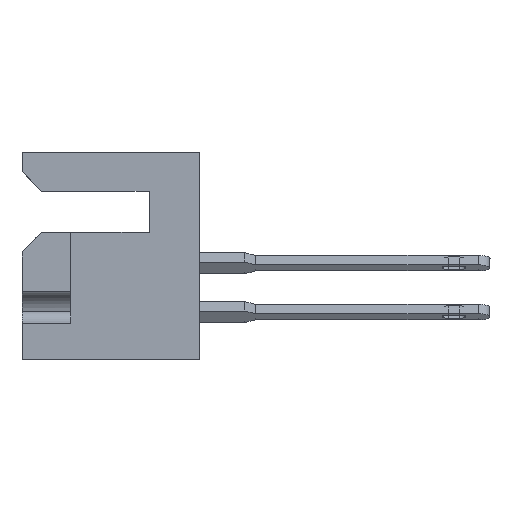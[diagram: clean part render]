
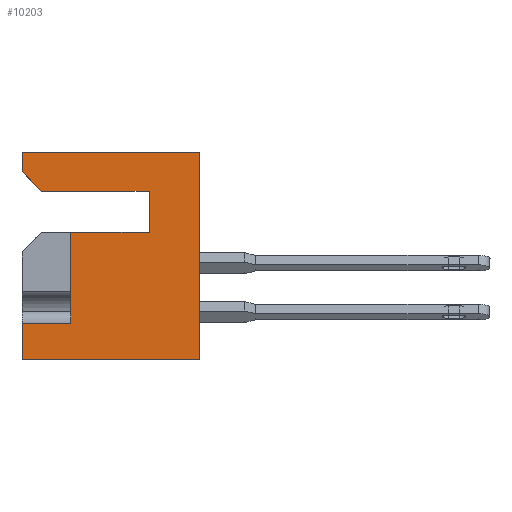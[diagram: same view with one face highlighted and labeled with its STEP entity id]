
A CAD part, left-side view. The second image highlights one B-rep face of the part: STEP entity #10203.
In plain terms, the highlighted planar face has unit normal (-1, 0, 0).
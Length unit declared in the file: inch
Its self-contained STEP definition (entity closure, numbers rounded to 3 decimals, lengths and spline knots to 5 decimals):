
#196 = VECTOR ( 'NONE', #16317, 39.37008 ) ;
#318 = DIRECTION ( 'NONE',  ( 0., -0.707, -0.707 ) ) ;
#600 = CARTESIAN_POINT ( 'NONE',  ( 0., 0.453, -0.437 ) ) ;
#619 = CARTESIAN_POINT ( 'NONE',  ( 0., 0.128, -0.1 ) ) ;
#1051 = DIRECTION ( 'NONE',  ( 0., 1., 0. ) ) ;
#1158 = ORIENTED_EDGE ( 'NONE', *, *, #29404, .F. ) ;
#1740 = EDGE_CURVE ( 'NONE', #29804, #2285, #30222, .T. ) ;
#2200 = EDGE_CURVE ( 'NONE', #2285, #3240, #10678, .T. ) ;
#2285 = VERTEX_POINT ( 'NONE', #9911 ) ;
#2516 = CARTESIAN_POINT ( 'NONE',  ( 0., 0.403, -0.1 ) ) ;
#2696 = LINE ( 'NONE', #619, #21012 ) ;
#3166 = DIRECTION ( 'NONE',  ( 0., 0., 1. ) ) ;
#3240 = VERTEX_POINT ( 'NONE', #20967 ) ;
#3398 = DIRECTION ( 'NONE',  ( 0., -1., 0. ) ) ;
#3488 = CARTESIAN_POINT ( 'NONE',  ( 0., 0.453, 0. ) ) ;
#3806 = ORIENTED_EDGE ( 'NONE', *, *, #1740, .T. ) ;
#4312 = CARTESIAN_POINT ( 'NONE',  ( 0., 0.453, -0.531 ) ) ;
#4360 = LINE ( 'NONE', #29978, #6949 ) ;
#5384 = CARTESIAN_POINT ( 'NONE',  ( 0., 0.453, -0.05 ) ) ;
#5457 = DIRECTION ( 'NONE',  ( 0., 0., 1. ) ) ;
#5610 = EDGE_CURVE ( 'NONE', #9739, #10014, #2696, .T. ) ;
#5795 = DIRECTION ( 'NONE',  ( 0., 1., 0. ) ) ;
#5845 = LINE ( 'NONE', #22413, #17781 ) ;
#6382 = EDGE_CURVE ( 'NONE', #22043, #27314, #6722, .T. ) ;
#6520 = LINE ( 'NONE', #18295, #196 ) ;
#6701 = CARTESIAN_POINT ( 'NONE',  ( 0., 0.128, -0.1 ) ) ;
#6722 = LINE ( 'NONE', #3488, #17491 ) ;
#6949 = VECTOR ( 'NONE', #1051, 39.37008 ) ;
#8115 = ORIENTED_EDGE ( 'NONE', *, *, #6382, .F. ) ;
#8143 = EDGE_CURVE ( 'NONE', #27314, #3240, #26451, .T. ) ;
#8195 = EDGE_CURVE ( 'NONE', #22358, #12789, #5845, .T. ) ;
#9115 = ORIENTED_EDGE ( 'NONE', *, *, #26209, .T. ) ;
#9739 = VERTEX_POINT ( 'NONE', #14934 ) ;
#9799 = DIRECTION ( 'NONE',  ( 0., 0., -1. ) ) ;
#9810 = CARTESIAN_POINT ( 'NONE',  ( 0., 0., 0. ) ) ;
#9911 = CARTESIAN_POINT ( 'NONE',  ( 0., 0., -0.531 ) ) ;
#10014 = VERTEX_POINT ( 'NONE', #6701 ) ;
#10203 = ADVANCED_FACE ( 'NONE', ( #15813 ), #17280, .F. ) ;
#10678 = LINE ( 'NONE', #9810, #23476 ) ;
#10777 = EDGE_CURVE ( 'NONE', #22043, #25842, #23697, .T. ) ;
#11663 = VECTOR ( 'NONE', #318, 39.37008 ) ;
#12358 = CARTESIAN_POINT ( 'NONE',  ( 0., 0.453, -0.531 ) ) ;
#12447 = ORIENTED_EDGE ( 'NONE', *, *, #5610, .F. ) ;
#12789 = VERTEX_POINT ( 'NONE', #17185 ) ;
#13010 = EDGE_CURVE ( 'NONE', #10014, #25842, #4360, .T. ) ;
#13811 = EDGE_CURVE ( 'NONE', #22358, #18755, #6520, .T. ) ;
#14658 = EDGE_LOOP ( 'NONE', ( #23924, #1158, #3806, #28747, #28792, #8115, #25415, #25661, #12447, #9115, #21869 ) ) ;
#14934 = CARTESIAN_POINT ( 'NONE',  ( 0., 0.128, -0.205 ) ) ;
#15813 = FACE_OUTER_BOUND ( 'NONE', #14658, .T. ) ;
#16317 = DIRECTION ( 'NONE',  ( 0., 1., 0. ) ) ;
#16990 = DIRECTION ( 'NONE',  ( 1., 0., 0. ) ) ;
#17185 = CARTESIAN_POINT ( 'NONE',  ( 0., 0.328, -0.205 ) ) ;
#17280 = PLANE ( 'NONE',  #22154 ) ;
#17491 = VECTOR ( 'NONE', #24609, 39.37008 ) ;
#17781 = VECTOR ( 'NONE', #17960, 39.37008 ) ;
#17811 = VECTOR ( 'NONE', #21823, 39.37008 ) ;
#17960 = DIRECTION ( 'NONE',  ( 0., 0., 1. ) ) ;
#18295 = CARTESIAN_POINT ( 'NONE',  ( 0., 0.328, -0.437 ) ) ;
#18755 = VERTEX_POINT ( 'NONE', #600 ) ;
#19410 = CARTESIAN_POINT ( 'NONE',  ( 0., 0.453, 0. ) ) ;
#20967 = CARTESIAN_POINT ( 'NONE',  ( 0., 0., 0. ) ) ;
#21012 = VECTOR ( 'NONE', #27244, 39.37008 ) ;
#21823 = DIRECTION ( 'NONE',  ( 0., -1., 0. ) ) ;
#21869 = ORIENTED_EDGE ( 'NONE', *, *, #8195, .F. ) ;
#21902 = LINE ( 'NONE', #25049, #27916 ) ;
#22043 = VERTEX_POINT ( 'NONE', #5384 ) ;
#22154 = AXIS2_PLACEMENT_3D ( 'NONE', #24266, #16990, #9799 ) ;
#22358 = VERTEX_POINT ( 'NONE', #23070 ) ;
#22413 = CARTESIAN_POINT ( 'NONE',  ( 0., 0.328, -0.205 ) ) ;
#23070 = CARTESIAN_POINT ( 'NONE',  ( 0., 0.328, -0.437 ) ) ;
#23415 = VECTOR ( 'NONE', #5457, 39.37008 ) ;
#23476 = VECTOR ( 'NONE', #3166, 39.37008 ) ;
#23697 = LINE ( 'NONE', #2516, #11663 ) ;
#23924 = ORIENTED_EDGE ( 'NONE', *, *, #13811, .T. ) ;
#24092 = CARTESIAN_POINT ( 'NONE',  ( 0., 0.453, 0. ) ) ;
#24266 = CARTESIAN_POINT ( 'NONE',  ( 0., 0.453, 0. ) ) ;
#24609 = DIRECTION ( 'NONE',  ( 0., 0., 1. ) ) ;
#25049 = CARTESIAN_POINT ( 'NONE',  ( 0., 0.128, -0.205 ) ) ;
#25381 = LINE ( 'NONE', #24092, #23415 ) ;
#25415 = ORIENTED_EDGE ( 'NONE', *, *, #10777, .T. ) ;
#25661 = ORIENTED_EDGE ( 'NONE', *, *, #13010, .F. ) ;
#25842 = VERTEX_POINT ( 'NONE', #28231 ) ;
#26209 = EDGE_CURVE ( 'NONE', #9739, #12789, #21902, .T. ) ;
#26451 = LINE ( 'NONE', #27119, #26804 ) ;
#26804 = VECTOR ( 'NONE', #3398, 39.37008 ) ;
#27119 = CARTESIAN_POINT ( 'NONE',  ( 0., 0.453, 0. ) ) ;
#27244 = DIRECTION ( 'NONE',  ( 0., 0., 1. ) ) ;
#27314 = VERTEX_POINT ( 'NONE', #19410 ) ;
#27916 = VECTOR ( 'NONE', #5795, 39.37008 ) ;
#28231 = CARTESIAN_POINT ( 'NONE',  ( 0., 0.403, -0.1 ) ) ;
#28747 = ORIENTED_EDGE ( 'NONE', *, *, #2200, .T. ) ;
#28792 = ORIENTED_EDGE ( 'NONE', *, *, #8143, .F. ) ;
#29404 = EDGE_CURVE ( 'NONE', #29804, #18755, #25381, .T. ) ;
#29804 = VERTEX_POINT ( 'NONE', #4312 ) ;
#29978 = CARTESIAN_POINT ( 'NONE',  ( 0., 0.128, -0.1 ) ) ;
#30222 = LINE ( 'NONE', #12358, #17811 ) ;
